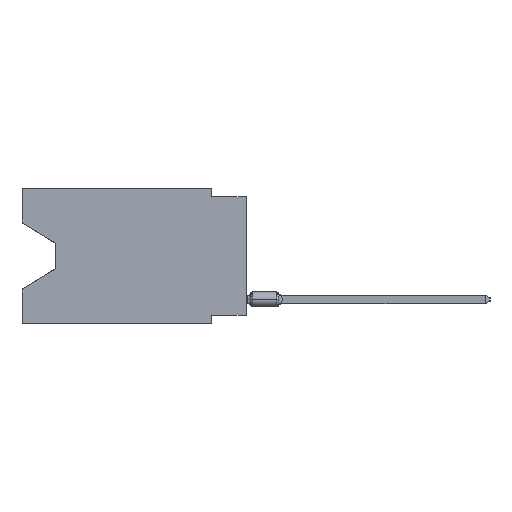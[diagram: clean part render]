
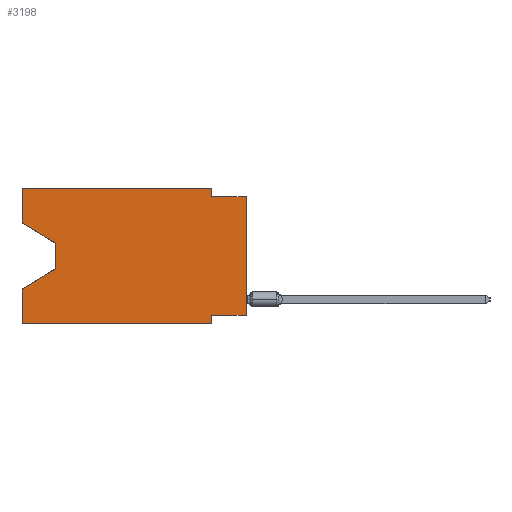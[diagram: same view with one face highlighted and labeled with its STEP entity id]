
A CAD part, left-side view. The second image highlights one B-rep face of the part: STEP entity #3198.
In plain terms, the highlighted planar face has unit normal (-1, 0, 0).
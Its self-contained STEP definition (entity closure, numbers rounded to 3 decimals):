
#412 = CARTESIAN_POINT ( 'NONE',  ( 0., 2.54, -0.635 ) ) ;
#766 = EDGE_CURVE ( 'NONE', #67937, #2094, #41665, .T. ) ;
#2094 = VERTEX_POINT ( 'NONE', #37736 ) ;
#2141 = CARTESIAN_POINT ( 'NONE',  ( 0., 0., -0.635 ) ) ;
#2503 = CARTESIAN_POINT ( 'NONE',  ( 0., 2.54, 0. ) ) ;
#2530 = DIRECTION ( 'NONE',  ( 0., -1., 0. ) ) ;
#3198 = ADVANCED_FACE ( 'NONE', ( #11744 ), #5117, .F. ) ;
#4350 = CARTESIAN_POINT ( 'NONE',  ( 0., 16.383, 0. ) ) ;
#4604 = VERTEX_POINT ( 'NONE', #12551 ) ;
#4814 = VERTEX_POINT ( 'NONE', #51879 ) ;
#4845 = EDGE_CURVE ( 'NONE', #2094, #33660, #58097, .T. ) ;
#5117 = PLANE ( 'NONE',  #28500 ) ;
#6141 = DIRECTION ( 'NONE',  ( 0., 1., 0. ) ) ;
#6591 = ORIENTED_EDGE ( 'NONE', *, *, #72686, .F. ) ;
#8569 = CARTESIAN_POINT ( 'NONE',  ( 0., 13.97, -4.013 ) ) ;
#8772 = LINE ( 'NONE', #2141, #51779 ) ;
#9356 = CARTESIAN_POINT ( 'NONE',  ( 0., 16.383, -2.546 ) ) ;
#11026 = VECTOR ( 'NONE', #17597, 1000. ) ;
#11744 = FACE_OUTER_BOUND ( 'NONE', #61158, .T. ) ;
#11844 = VECTOR ( 'NONE', #6141, 1000. ) ;
#12230 = VECTOR ( 'NONE', #51485, 1000. ) ;
#12551 = CARTESIAN_POINT ( 'NONE',  ( 0., 2.54, 0. ) ) ;
#14044 = ORIENTED_EDGE ( 'NONE', *, *, #71822, .T. ) ;
#14594 = VECTOR ( 'NONE', #43657, 1000. ) ;
#14884 = VECTOR ( 'NONE', #66801, 1000. ) ;
#15768 = DIRECTION ( 'NONE',  ( 0., 0., -1. ) ) ;
#16780 = DIRECTION ( 'NONE',  ( 0., -0.855, -0.519 ) ) ;
#17597 = DIRECTION ( 'NONE',  ( 0., 0., 1. ) ) ;
#19212 = LINE ( 'NONE', #43000, #14884 ) ;
#19965 = CARTESIAN_POINT ( 'NONE',  ( 0., 16.383, -9.906 ) ) ;
#23046 = CARTESIAN_POINT ( 'NONE',  ( 0., 16.383, 0. ) ) ;
#23316 = VECTOR ( 'NONE', #68384, 1000. ) ;
#23772 = VECTOR ( 'NONE', #75689, 1000. ) ;
#25649 = EDGE_CURVE ( 'NONE', #50297, #33660, #48332, .T. ) ;
#26388 = CARTESIAN_POINT ( 'NONE',  ( 0., 2.54, -9.906 ) ) ;
#27392 = DIRECTION ( 'NONE',  ( 0., 0.855, -0.519 ) ) ;
#28500 = AXIS2_PLACEMENT_3D ( 'NONE', #4350, #35540, #51947 ) ;
#30435 = VECTOR ( 'NONE', #27392, 1000. ) ;
#30469 = EDGE_CURVE ( 'NONE', #50962, #51976, #46825, .T. ) ;
#31187 = CARTESIAN_POINT ( 'NONE',  ( 0., 16.383, -9.906 ) ) ;
#31337 = CARTESIAN_POINT ( 'NONE',  ( 0., 0., 0. ) ) ;
#33149 = LINE ( 'NONE', #8569, #12230 ) ;
#33247 = CARTESIAN_POINT ( 'NONE',  ( 0., 13.97, -5.893 ) ) ;
#33254 = EDGE_CURVE ( 'NONE', #50297, #71022, #19212, .T. ) ;
#33660 = VERTEX_POINT ( 'NONE', #26388 ) ;
#34454 = ORIENTED_EDGE ( 'NONE', *, *, #33254, .F. ) ;
#35540 = DIRECTION ( 'NONE',  ( 1., 0., 0. ) ) ;
#37180 = LINE ( 'NONE', #31337, #23316 ) ;
#37736 = CARTESIAN_POINT ( 'NONE',  ( 0., 2.54, -9.271 ) ) ;
#39972 = CARTESIAN_POINT ( 'NONE',  ( 0., 16.383, -7.36 ) ) ;
#41665 = LINE ( 'NONE', #77161, #11844 ) ;
#42710 = ORIENTED_EDGE ( 'NONE', *, *, #25649, .T. ) ;
#43000 = CARTESIAN_POINT ( 'NONE',  ( 0., 16.383, 0. ) ) ;
#43657 = DIRECTION ( 'NONE',  ( 0., -1., 0. ) ) ;
#44398 = VERTEX_POINT ( 'NONE', #33247 ) ;
#44882 = CARTESIAN_POINT ( 'NONE',  ( 0., 2.54, -9.906 ) ) ;
#44946 = LINE ( 'NONE', #62520, #30435 ) ;
#45275 = CARTESIAN_POINT ( 'NONE',  ( 0., 13.97, -4.013 ) ) ;
#45885 = ORIENTED_EDGE ( 'NONE', *, *, #52292, .F. ) ;
#46825 = LINE ( 'NONE', #23046, #11026 ) ;
#47199 = VERTEX_POINT ( 'NONE', #412 ) ;
#48332 = LINE ( 'NONE', #31187, #14594 ) ;
#48663 = VECTOR ( 'NONE', #16780, 1000. ) ;
#50069 = ORIENTED_EDGE ( 'NONE', *, *, #59468, .F. ) ;
#50297 = VERTEX_POINT ( 'NONE', #19965 ) ;
#50962 = VERTEX_POINT ( 'NONE', #62969 ) ;
#51121 = DIRECTION ( 'NONE',  ( 0., 0., -1. ) ) ;
#51485 = DIRECTION ( 'NONE',  ( 0., 0., -1. ) ) ;
#51779 = VECTOR ( 'NONE', #2530, 1000. ) ;
#51879 = CARTESIAN_POINT ( 'NONE',  ( 0., 0., -0.635 ) ) ;
#51947 = DIRECTION ( 'NONE',  ( 0., 0., -1. ) ) ;
#51976 = VERTEX_POINT ( 'NONE', #76031 ) ;
#52292 = EDGE_CURVE ( 'NONE', #4604, #47199, #55943, .T. ) ;
#54550 = EDGE_CURVE ( 'NONE', #44398, #71022, #44946, .T. ) ;
#54859 = ORIENTED_EDGE ( 'NONE', *, *, #30469, .F. ) ;
#55735 = ORIENTED_EDGE ( 'NONE', *, *, #766, .F. ) ;
#55943 = LINE ( 'NONE', #2503, #73835 ) ;
#57724 = LINE ( 'NONE', #64345, #23772 ) ;
#58097 = LINE ( 'NONE', #44882, #59655 ) ;
#59468 = EDGE_CURVE ( 'NONE', #51976, #4604, #57724, .T. ) ;
#59602 = EDGE_CURVE ( 'NONE', #50962, #61140, #70223, .T. ) ;
#59655 = VECTOR ( 'NONE', #51121, 1000. ) ;
#60664 = CARTESIAN_POINT ( 'NONE',  ( 0., 0., -9.271 ) ) ;
#61140 = VERTEX_POINT ( 'NONE', #45275 ) ;
#61158 = EDGE_LOOP ( 'NONE', ( #71698, #14044, #69686, #34454, #42710, #76832, #55735, #71885, #6591, #45885, #50069, #54859 ) ) ;
#62520 = CARTESIAN_POINT ( 'NONE',  ( 0., 13.97, -5.893 ) ) ;
#62969 = CARTESIAN_POINT ( 'NONE',  ( 0., 16.383, -2.546 ) ) ;
#64345 = CARTESIAN_POINT ( 'NONE',  ( 0., 16.383, 0. ) ) ;
#66801 = DIRECTION ( 'NONE',  ( 0., 0., 1. ) ) ;
#67937 = VERTEX_POINT ( 'NONE', #60664 ) ;
#68384 = DIRECTION ( 'NONE',  ( 0., 0., 1. ) ) ;
#69686 = ORIENTED_EDGE ( 'NONE', *, *, #54550, .T. ) ;
#70223 = LINE ( 'NONE', #9356, #48663 ) ;
#71022 = VERTEX_POINT ( 'NONE', #39972 ) ;
#71698 = ORIENTED_EDGE ( 'NONE', *, *, #59602, .T. ) ;
#71822 = EDGE_CURVE ( 'NONE', #61140, #44398, #33149, .T. ) ;
#71885 = ORIENTED_EDGE ( 'NONE', *, *, #74234, .T. ) ;
#72686 = EDGE_CURVE ( 'NONE', #47199, #4814, #8772, .T. ) ;
#73835 = VECTOR ( 'NONE', #15768, 1000. ) ;
#74234 = EDGE_CURVE ( 'NONE', #67937, #4814, #37180, .T. ) ;
#75689 = DIRECTION ( 'NONE',  ( 0., -1., 0. ) ) ;
#76031 = CARTESIAN_POINT ( 'NONE',  ( 0., 16.383, 0. ) ) ;
#76832 = ORIENTED_EDGE ( 'NONE', *, *, #4845, .F. ) ;
#77161 = CARTESIAN_POINT ( 'NONE',  ( 0., 0., -9.271 ) ) ;
